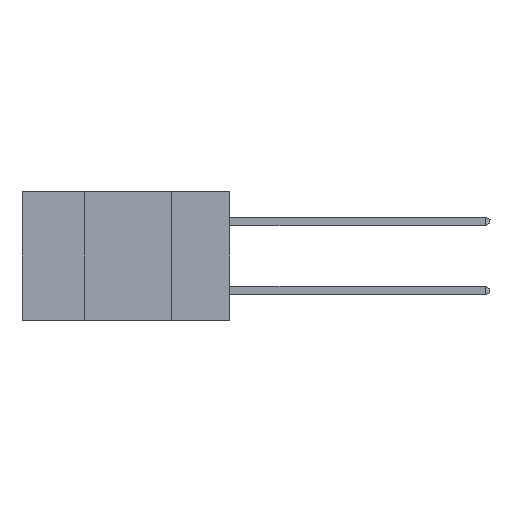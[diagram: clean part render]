
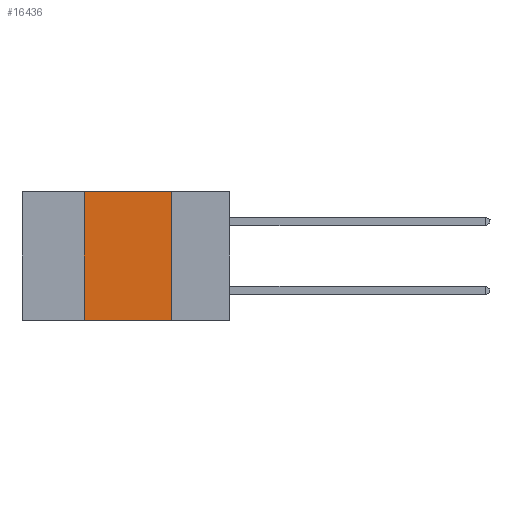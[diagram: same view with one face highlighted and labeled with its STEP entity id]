
A CAD part, left-side view. The second image highlights one B-rep face of the part: STEP entity #16436.
In plain terms, the highlighted planar face has unit normal (-1, 0, 0).
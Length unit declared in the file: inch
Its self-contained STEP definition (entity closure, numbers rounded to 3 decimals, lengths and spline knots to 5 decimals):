
#123 = VECTOR ( 'NONE', #5089, 39.37008 ) ;
#1101 = LINE ( 'NONE', #13479, #3417 ) ;
#1159 = ORIENTED_EDGE ( 'NONE', *, *, #6977, .F. ) ;
#1296 = ORIENTED_EDGE ( 'NONE', *, *, #8367, .T. ) ;
#2077 = DIRECTION ( 'NONE',  ( 0., 0., -1. ) ) ;
#2237 = CARTESIAN_POINT ( 'NONE',  ( 0., 0.42, 0. ) ) ;
#2298 = CARTESIAN_POINT ( 'NONE',  ( 0., 0.17, -0.37 ) ) ;
#2577 = CARTESIAN_POINT ( 'NONE',  ( 0., 0.6, 0. ) ) ;
#3228 = LINE ( 'NONE', #16618, #7605 ) ;
#3417 = VECTOR ( 'NONE', #10538, 39.37008 ) ;
#3814 = VECTOR ( 'NONE', #10994, 39.37008 ) ;
#3847 = ORIENTED_EDGE ( 'NONE', *, *, #13403, .F. ) ;
#5089 = DIRECTION ( 'NONE',  ( 0., 0., -1. ) ) ;
#6977 = EDGE_CURVE ( 'NONE', #12361, #13015, #1101, .T. ) ;
#7540 = CARTESIAN_POINT ( 'NONE',  ( 0., 0.17, -0.37 ) ) ;
#7605 = VECTOR ( 'NONE', #12715, 39.37008 ) ;
#8123 = VERTEX_POINT ( 'NONE', #12996 ) ;
#8367 = EDGE_CURVE ( 'NONE', #12361, #14336, #3228, .T. ) ;
#8724 = CARTESIAN_POINT ( 'NONE',  ( 0., 0.42, -0.37 ) ) ;
#8908 = DIRECTION ( 'NONE',  ( 1., 0., 0. ) ) ;
#9349 = ORIENTED_EDGE ( 'NONE', *, *, #10423, .F. ) ;
#9809 = FACE_OUTER_BOUND ( 'NONE', #10958, .T. ) ;
#10361 = LINE ( 'NONE', #2298, #123 ) ;
#10423 = EDGE_CURVE ( 'NONE', #13015, #8123, #12147, .T. ) ;
#10538 = DIRECTION ( 'NONE',  ( 0., 0., 1. ) ) ;
#10958 = EDGE_LOOP ( 'NONE', ( #3847, #9349, #1159, #1296 ) ) ;
#10994 = DIRECTION ( 'NONE',  ( 0., -1., 0. ) ) ;
#11080 = AXIS2_PLACEMENT_3D ( 'NONE', #11749, #8908, #2077 ) ;
#11749 = CARTESIAN_POINT ( 'NONE',  ( 0., 0.6, 0. ) ) ;
#12147 = LINE ( 'NONE', #2577, #3814 ) ;
#12361 = VERTEX_POINT ( 'NONE', #8724 ) ;
#12715 = DIRECTION ( 'NONE',  ( 0., -1., 0. ) ) ;
#12996 = CARTESIAN_POINT ( 'NONE',  ( 0., 0.17, 0. ) ) ;
#13015 = VERTEX_POINT ( 'NONE', #2237 ) ;
#13403 = EDGE_CURVE ( 'NONE', #8123, #14336, #10361, .T. ) ;
#13479 = CARTESIAN_POINT ( 'NONE',  ( 0., 0.42, -0.37 ) ) ;
#14336 = VERTEX_POINT ( 'NONE', #7540 ) ;
#15274 = PLANE ( 'NONE',  #11080 ) ;
#16436 = ADVANCED_FACE ( 'NONE', ( #9809 ), #15274, .F. ) ;
#16618 = CARTESIAN_POINT ( 'NONE',  ( 0., 0.6, -0.37 ) ) ;
